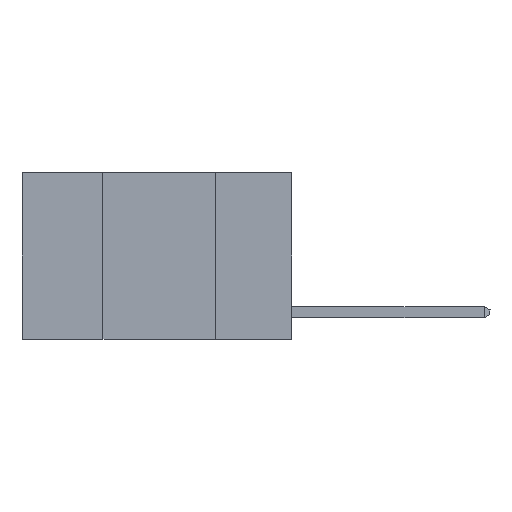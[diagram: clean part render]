
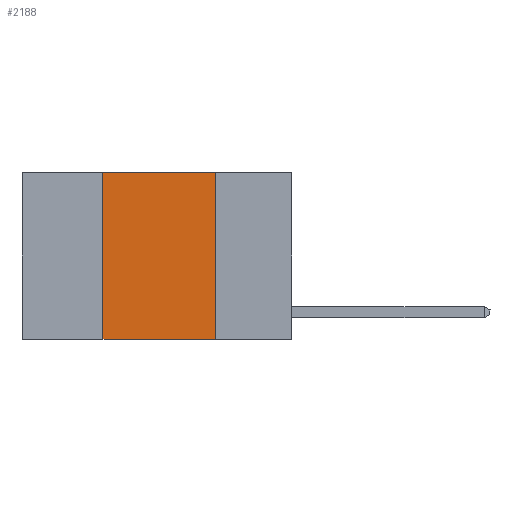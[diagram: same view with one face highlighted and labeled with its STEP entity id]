
A CAD part, left-side view. The second image highlights one B-rep face of the part: STEP entity #2188.
In plain terms, the highlighted planar face has unit normal (-1, 0, 0).
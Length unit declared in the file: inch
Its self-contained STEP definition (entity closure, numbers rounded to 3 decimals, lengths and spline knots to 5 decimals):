
#1105 = CARTESIAN_POINT ( 'NONE',  ( 0., 0.6, 0. ) ) ;
#1742 = CARTESIAN_POINT ( 'NONE',  ( 0., 0.6, -0.37 ) ) ;
#1766 = ORIENTED_EDGE ( 'NONE', *, *, #11474, .T. ) ;
#1860 = DIRECTION ( 'NONE',  ( 0., -1., 0. ) ) ;
#1972 = CARTESIAN_POINT ( 'NONE',  ( 0., 0.6, 0. ) ) ;
#2188 = ADVANCED_FACE ( 'NONE', ( #7002 ), #6328, .F. ) ;
#2649 = EDGE_CURVE ( 'NONE', #7748, #13321, #15203, .T. ) ;
#3086 = VECTOR ( 'NONE', #13766, 39.37008 ) ;
#3167 = CARTESIAN_POINT ( 'NONE',  ( 0., 0.17, 0. ) ) ;
#4449 = EDGE_CURVE ( 'NONE', #13321, #16081, #13340, .T. ) ;
#5485 = DIRECTION ( 'NONE',  ( 0., 0., -1. ) ) ;
#5581 = DIRECTION ( 'NONE',  ( 0., 0., 1. ) ) ;
#6095 = VERTEX_POINT ( 'NONE', #9653 ) ;
#6328 = PLANE ( 'NONE',  #16260 ) ;
#6794 = CARTESIAN_POINT ( 'NONE',  ( 0., 0.42, -0.37 ) ) ;
#7002 = FACE_OUTER_BOUND ( 'NONE', #12561, .T. ) ;
#7748 = VERTEX_POINT ( 'NONE', #6794 ) ;
#8226 = VECTOR ( 'NONE', #1860, 39.37008 ) ;
#9653 = CARTESIAN_POINT ( 'NONE',  ( 0., 0.17, -0.37 ) ) ;
#9858 = ORIENTED_EDGE ( 'NONE', *, *, #4449, .F. ) ;
#10940 = EDGE_CURVE ( 'NONE', #16081, #6095, #14548, .T. ) ;
#11082 = CARTESIAN_POINT ( 'NONE',  ( 0., 0.42, 0. ) ) ;
#11276 = DIRECTION ( 'NONE',  ( 0., -1., 0. ) ) ;
#11474 = EDGE_CURVE ( 'NONE', #7748, #6095, #11659, .T. ) ;
#11659 = LINE ( 'NONE', #1742, #8226 ) ;
#12181 = CARTESIAN_POINT ( 'NONE',  ( 0., 0.42, 0. ) ) ;
#12561 = EDGE_LOOP ( 'NONE', ( #15448, #9858, #13967, #1766 ) ) ;
#13321 = VERTEX_POINT ( 'NONE', #11082 ) ;
#13340 = LINE ( 'NONE', #1972, #15189 ) ;
#13766 = DIRECTION ( 'NONE',  ( 0., 0., -1. ) ) ;
#13967 = ORIENTED_EDGE ( 'NONE', *, *, #2649, .F. ) ;
#14375 = VECTOR ( 'NONE', #5581, 39.37008 ) ;
#14548 = LINE ( 'NONE', #14962, #3086 ) ;
#14962 = CARTESIAN_POINT ( 'NONE',  ( 0., 0.17, 0. ) ) ;
#15189 = VECTOR ( 'NONE', #11276, 39.37008 ) ;
#15203 = LINE ( 'NONE', #12181, #14375 ) ;
#15448 = ORIENTED_EDGE ( 'NONE', *, *, #10940, .F. ) ;
#15892 = DIRECTION ( 'NONE',  ( 1., 0., 0. ) ) ;
#16081 = VERTEX_POINT ( 'NONE', #3167 ) ;
#16260 = AXIS2_PLACEMENT_3D ( 'NONE', #1105, #15892, #5485 ) ;
